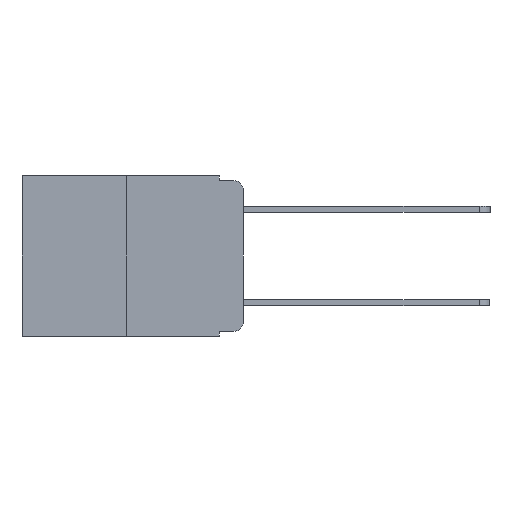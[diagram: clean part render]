
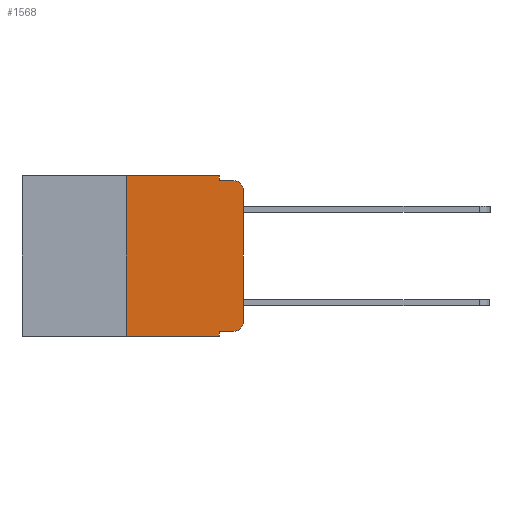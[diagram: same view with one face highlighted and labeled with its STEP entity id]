
A CAD part, left-side view. The second image highlights one B-rep face of the part: STEP entity #1568.
In plain terms, the highlighted planar face has unit normal (-1, 0, 0).
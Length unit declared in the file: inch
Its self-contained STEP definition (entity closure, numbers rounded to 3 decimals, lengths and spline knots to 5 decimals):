
#50 = FACE_OUTER_BOUND ( 'NONE', #8410, .T. ) ;
#152 = VECTOR ( 'NONE', #504, 39.37008 ) ;
#189 = VECTOR ( 'NONE', #10535, 39.37008 ) ;
#414 = CARTESIAN_POINT ( 'NONE',  ( 0., 0.051, -0.01 ) ) ;
#449 = VECTOR ( 'NONE', #549, 39.37008 ) ;
#486 = PLANE ( 'NONE',  #10413 ) ;
#497 = VERTEX_POINT ( 'NONE', #10677 ) ;
#504 = DIRECTION ( 'NONE',  ( 0., -1., 0. ) ) ;
#549 = DIRECTION ( 'NONE',  ( 0., 0., 1. ) ) ;
#573 = DIRECTION ( 'NONE',  ( -1., 0., 0. ) ) ;
#583 = CARTESIAN_POINT ( 'NONE',  ( 0., 0.02, -0.313 ) ) ;
#644 = DIRECTION ( 'NONE',  ( -1., 0., 0. ) ) ;
#670 = DIRECTION ( 'NONE',  ( 0., 0., -1. ) ) ;
#763 = CARTESIAN_POINT ( 'NONE',  ( 0., 0., -0.03 ) ) ;
#804 = CARTESIAN_POINT ( 'NONE',  ( 0., 0.02, -0.333 ) ) ;
#838 = CARTESIAN_POINT ( 'NONE',  ( 0., 0.25, 0. ) ) ;
#852 = LINE ( 'NONE', #4610, #2911 ) ;
#871 = CARTESIAN_POINT ( 'NONE',  ( 0., 0.051, -0.333 ) ) ;
#1451 = CARTESIAN_POINT ( 'NONE',  ( 0., 0.051, 0. ) ) ;
#1568 = ADVANCED_FACE ( 'NONE', ( #50 ), #486, .F. ) ;
#1725 = DIRECTION ( 'NONE',  ( 0., -1., 0. ) ) ;
#1729 = CARTESIAN_POINT ( 'NONE',  ( 0., 0.473, 0. ) ) ;
#2079 = ORIENTED_EDGE ( 'NONE', *, *, #3308, .F. ) ;
#2218 = ORIENTED_EDGE ( 'NONE', *, *, #3039, .T. ) ;
#2242 = ORIENTED_EDGE ( 'NONE', *, *, #4424, .F. ) ;
#2349 = EDGE_CURVE ( 'NONE', #3713, #497, #4938, .T. ) ;
#2412 = AXIS2_PLACEMENT_3D ( 'NONE', #5973, #644, #6834 ) ;
#2471 = DIRECTION ( 'NONE',  ( 0., 0., -1. ) ) ;
#2505 = EDGE_CURVE ( 'NONE', #9976, #8295, #3225, .T. ) ;
#2530 = ORIENTED_EDGE ( 'NONE', *, *, #6305, .F. ) ;
#2631 = ORIENTED_EDGE ( 'NONE', *, *, #2505, .F. ) ;
#2761 = CARTESIAN_POINT ( 'NONE',  ( 0., 0.02, -0.01 ) ) ;
#2911 = VECTOR ( 'NONE', #9626, 39.37008 ) ;
#2973 = ORIENTED_EDGE ( 'NONE', *, *, #6733, .T. ) ;
#3039 = EDGE_CURVE ( 'NONE', #3329, #497, #6825, .T. ) ;
#3125 = LINE ( 'NONE', #871, #9693 ) ;
#3225 = LINE ( 'NONE', #9387, #8097 ) ;
#3308 = EDGE_CURVE ( 'NONE', #3329, #6580, #8852, .T. ) ;
#3329 = VERTEX_POINT ( 'NONE', #3469 ) ;
#3333 = ORIENTED_EDGE ( 'NONE', *, *, #7618, .T. ) ;
#3469 = CARTESIAN_POINT ( 'NONE',  ( 0., 0.25, -0.343 ) ) ;
#3712 = EDGE_CURVE ( 'NONE', #6889, #10131, #9619, .T. ) ;
#3713 = VERTEX_POINT ( 'NONE', #7671 ) ;
#3818 = DIRECTION ( 'NONE',  ( 0., -1., 0. ) ) ;
#4238 = AXIS2_PLACEMENT_3D ( 'NONE', #583, #573, #670 ) ;
#4424 = EDGE_CURVE ( 'NONE', #6580, #9976, #5302, .T. ) ;
#4518 = VECTOR ( 'NONE', #3818, 39.37008 ) ;
#4610 = CARTESIAN_POINT ( 'NONE',  ( 0., 0., 0. ) ) ;
#4938 = LINE ( 'NONE', #9479, #189 ) ;
#5026 = VECTOR ( 'NONE', #7310, 39.37008 ) ;
#5168 = CIRCLE ( 'NONE', #2412, 0.02 ) ;
#5302 = LINE ( 'NONE', #10067, #5026 ) ;
#5448 = ORIENTED_EDGE ( 'NONE', *, *, #3712, .T. ) ;
#5464 = LINE ( 'NONE', #9852, #152 ) ;
#5483 = ORIENTED_EDGE ( 'NONE', *, *, #2349, .F. ) ;
#5967 = CARTESIAN_POINT ( 'NONE',  ( 0., 0.25, 0. ) ) ;
#5973 = CARTESIAN_POINT ( 'NONE',  ( 0., 0.02, -0.03 ) ) ;
#6305 = EDGE_CURVE ( 'NONE', #8295, #10261, #5464, .T. ) ;
#6580 = VERTEX_POINT ( 'NONE', #838 ) ;
#6733 = EDGE_CURVE ( 'NONE', #6819, #10261, #5168, .T. ) ;
#6819 = VERTEX_POINT ( 'NONE', #763 ) ;
#6825 = LINE ( 'NONE', #10608, #4518 ) ;
#6834 = DIRECTION ( 'NONE',  ( 0., 0., -1. ) ) ;
#6889 = VERTEX_POINT ( 'NONE', #804 ) ;
#6978 = CARTESIAN_POINT ( 'NONE',  ( 0., 0., -0.313 ) ) ;
#7310 = DIRECTION ( 'NONE',  ( 0., -1., 0. ) ) ;
#7599 = DIRECTION ( 'NONE',  ( 0., 0., -1. ) ) ;
#7618 = EDGE_CURVE ( 'NONE', #10131, #6819, #852, .T. ) ;
#7671 = CARTESIAN_POINT ( 'NONE',  ( 0., 0.051, -0.333 ) ) ;
#8097 = VECTOR ( 'NONE', #2471, 39.37008 ) ;
#8295 = VERTEX_POINT ( 'NONE', #414 ) ;
#8410 = EDGE_LOOP ( 'NONE', ( #3333, #2973, #2530, #2631, #2242, #2079, #2218, #5483, #8558, #5448 ) ) ;
#8558 = ORIENTED_EDGE ( 'NONE', *, *, #9258, .T. ) ;
#8852 = LINE ( 'NONE', #5967, #449 ) ;
#9258 = EDGE_CURVE ( 'NONE', #3713, #6889, #3125, .T. ) ;
#9387 = CARTESIAN_POINT ( 'NONE',  ( 0., 0.051, 0. ) ) ;
#9412 = DIRECTION ( 'NONE',  ( 1., 0., 0. ) ) ;
#9479 = CARTESIAN_POINT ( 'NONE',  ( 0., 0.051, 0. ) ) ;
#9619 = CIRCLE ( 'NONE', #4238, 0.02 ) ;
#9626 = DIRECTION ( 'NONE',  ( 0., 0., 1. ) ) ;
#9693 = VECTOR ( 'NONE', #1725, 39.37008 ) ;
#9852 = CARTESIAN_POINT ( 'NONE',  ( 0., 0.051, -0.01 ) ) ;
#9976 = VERTEX_POINT ( 'NONE', #1451 ) ;
#10067 = CARTESIAN_POINT ( 'NONE',  ( 0., 0.473, 0. ) ) ;
#10131 = VERTEX_POINT ( 'NONE', #6978 ) ;
#10261 = VERTEX_POINT ( 'NONE', #2761 ) ;
#10413 = AXIS2_PLACEMENT_3D ( 'NONE', #1729, #9412, #7599 ) ;
#10535 = DIRECTION ( 'NONE',  ( 0., 0., -1. ) ) ;
#10608 = CARTESIAN_POINT ( 'NONE',  ( 0., 0.473, -0.343 ) ) ;
#10677 = CARTESIAN_POINT ( 'NONE',  ( 0., 0.051, -0.343 ) ) ;
